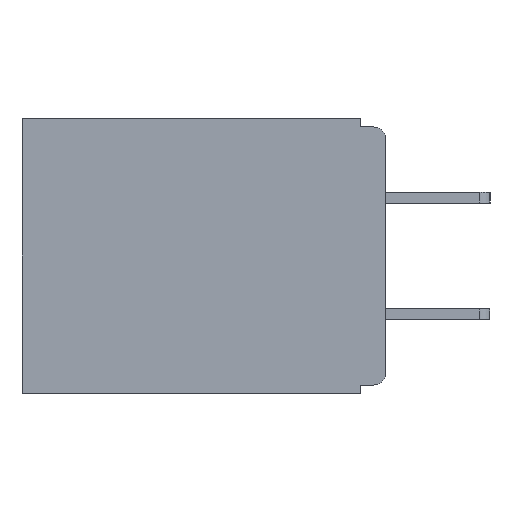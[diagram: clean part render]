
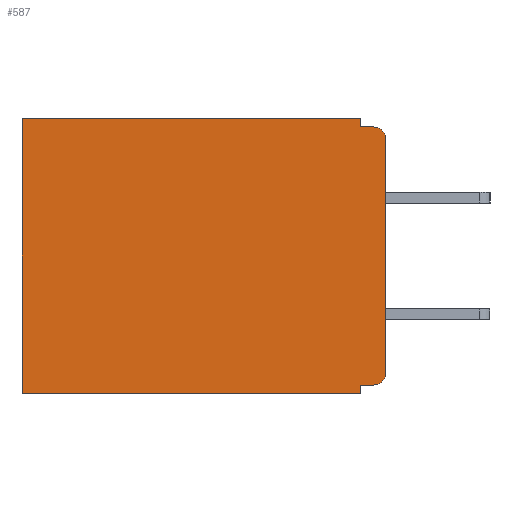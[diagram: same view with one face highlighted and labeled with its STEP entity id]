
A CAD part, left-side view. The second image highlights one B-rep face of the part: STEP entity #587.
In plain terms, the highlighted planar face has unit normal (-1, 0, 0).
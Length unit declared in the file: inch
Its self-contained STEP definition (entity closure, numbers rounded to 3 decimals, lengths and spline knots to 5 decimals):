
#24 = ORIENTED_EDGE ( 'NONE', *, *, #12456, .T. ) ;
#113 = EDGE_CURVE ( 'NONE', #2169, #9449, #17951, .T. ) ;
#400 = AXIS2_PLACEMENT_3D ( 'NONE', #11541, #19449, #19318 ) ;
#406 = CARTESIAN_POINT ( 'NONE',  ( 0.3, 0.031, 0. ) ) ;
#587 = ADVANCED_FACE ( 'NONE', ( #16894 ), #5696, .F. ) ;
#674 = LINE ( 'NONE', #2899, #17898 ) ;
#860 = VECTOR ( 'NONE', #5412, 39.37008 ) ;
#1231 = ORIENTED_EDGE ( 'NONE', *, *, #1955, .F. ) ;
#1410 = CARTESIAN_POINT ( 'NONE',  ( 0.3, 0.031, -0.01 ) ) ;
#1955 = EDGE_CURVE ( 'NONE', #13222, #3481, #2983, .T. ) ;
#2047 = CARTESIAN_POINT ( 'NONE',  ( 0.3, 0.031, -0.33 ) ) ;
#2169 = VERTEX_POINT ( 'NONE', #2966 ) ;
#2665 = CARTESIAN_POINT ( 'NONE',  ( 0.3, 0., -0.305 ) ) ;
#2899 = CARTESIAN_POINT ( 'NONE',  ( 0.3, 0., 0. ) ) ;
#2966 = CARTESIAN_POINT ( 'NONE',  ( 0.3, 0., -0.025 ) ) ;
#2983 = LINE ( 'NONE', #6736, #20175 ) ;
#3008 = ORIENTED_EDGE ( 'NONE', *, *, #3570, .T. ) ;
#3139 = EDGE_CURVE ( 'NONE', #14326, #16589, #4849, .T. ) ;
#3334 = DIRECTION ( 'NONE',  ( -1., 0., 0. ) ) ;
#3481 = VERTEX_POINT ( 'NONE', #20053 ) ;
#3570 = EDGE_CURVE ( 'NONE', #2169, #16589, #9251, .T. ) ;
#4005 = EDGE_CURVE ( 'NONE', #12849, #9449, #9772, .T. ) ;
#4008 = VECTOR ( 'NONE', #18722, 39.37008 ) ;
#4676 = VERTEX_POINT ( 'NONE', #406 ) ;
#4700 = EDGE_CURVE ( 'NONE', #18115, #13222, #18253, .T. ) ;
#4849 = LINE ( 'NONE', #18784, #9819 ) ;
#5397 = LINE ( 'NONE', #11966, #860 ) ;
#5410 = ORIENTED_EDGE ( 'NONE', *, *, #9202, .F. ) ;
#5412 = DIRECTION ( 'NONE',  ( 0., 0., -1. ) ) ;
#5484 = CARTESIAN_POINT ( 'NONE',  ( 0.3, 0., -0.32 ) ) ;
#5696 = PLANE ( 'NONE',  #400 ) ;
#6101 = ORIENTED_EDGE ( 'NONE', *, *, #3139, .F. ) ;
#6109 = CARTESIAN_POINT ( 'NONE',  ( 0.3, 0.015, -0.32 ) ) ;
#6736 = CARTESIAN_POINT ( 'NONE',  ( 0.3, 0., -0.33 ) ) ;
#6982 = EDGE_LOOP ( 'NONE', ( #16431, #3008, #6101, #16117, #24, #18254, #1231, #18808, #5410, #8944 ) ) ;
#7093 = CARTESIAN_POINT ( 'NONE',  ( 0.3, 0.031, -0.32 ) ) ;
#7620 = DIRECTION ( 'NONE',  ( -1., 0., 0. ) ) ;
#7667 = CARTESIAN_POINT ( 'NONE',  ( 0.3, 0.015, -0.305 ) ) ;
#7770 = CARTESIAN_POINT ( 'NONE',  ( 0.3, 0.015, -0.01 ) ) ;
#8492 = LINE ( 'NONE', #5484, #4008 ) ;
#8944 = ORIENTED_EDGE ( 'NONE', *, *, #4005, .T. ) ;
#9101 = EDGE_CURVE ( 'NONE', #18531, #3481, #19645, .T. ) ;
#9168 = EDGE_CURVE ( 'NONE', #4676, #14326, #5397, .T. ) ;
#9202 = EDGE_CURVE ( 'NONE', #12849, #18115, #8492, .T. ) ;
#9251 = CIRCLE ( 'NONE', #21141, 0.015 ) ;
#9449 = VERTEX_POINT ( 'NONE', #2665 ) ;
#9458 = CARTESIAN_POINT ( 'NONE',  ( 0.3, 0.015, -0.025 ) ) ;
#9686 = VECTOR ( 'NONE', #12217, 39.37008 ) ;
#9770 = DIRECTION ( 'NONE',  ( 0., 1., 0. ) ) ;
#9772 = CIRCLE ( 'NONE', #19671, 0.015 ) ;
#9819 = VECTOR ( 'NONE', #10908, 39.37008 ) ;
#10908 = DIRECTION ( 'NONE',  ( 0., -1., 0. ) ) ;
#11541 = CARTESIAN_POINT ( 'NONE',  ( 0.3, 0., -0.33 ) ) ;
#11760 = CARTESIAN_POINT ( 'NONE',  ( 0.3, 0.437, -0.33 ) ) ;
#11966 = CARTESIAN_POINT ( 'NONE',  ( 0.3, 0.031, 0. ) ) ;
#12217 = DIRECTION ( 'NONE',  ( 0., 0., -1. ) ) ;
#12286 = CARTESIAN_POINT ( 'NONE',  ( 0.3, 0., -0.33 ) ) ;
#12456 = EDGE_CURVE ( 'NONE', #4676, #18531, #674, .T. ) ;
#12789 = DIRECTION ( 'NONE',  ( 0., 1., 0. ) ) ;
#12849 = VERTEX_POINT ( 'NONE', #6109 ) ;
#13130 = CARTESIAN_POINT ( 'NONE',  ( 0.3, 0.437, 0. ) ) ;
#13222 = VERTEX_POINT ( 'NONE', #2047 ) ;
#13839 = VECTOR ( 'NONE', #21049, 39.37008 ) ;
#14326 = VERTEX_POINT ( 'NONE', #1410 ) ;
#15230 = VECTOR ( 'NONE', #16784, 39.37008 ) ;
#15950 = DIRECTION ( 'NONE',  ( 0., 0., -1. ) ) ;
#16117 = ORIENTED_EDGE ( 'NONE', *, *, #9168, .F. ) ;
#16431 = ORIENTED_EDGE ( 'NONE', *, *, #113, .F. ) ;
#16589 = VERTEX_POINT ( 'NONE', #7770 ) ;
#16718 = DIRECTION ( 'NONE',  ( 0., 0., -1. ) ) ;
#16784 = DIRECTION ( 'NONE',  ( 0., 0., -1. ) ) ;
#16894 = FACE_OUTER_BOUND ( 'NONE', #6982, .T. ) ;
#17898 = VECTOR ( 'NONE', #9770, 39.37008 ) ;
#17951 = LINE ( 'NONE', #12286, #9686 ) ;
#18115 = VERTEX_POINT ( 'NONE', #7093 ) ;
#18253 = LINE ( 'NONE', #18883, #13839 ) ;
#18254 = ORIENTED_EDGE ( 'NONE', *, *, #9101, .T. ) ;
#18531 = VERTEX_POINT ( 'NONE', #13130 ) ;
#18722 = DIRECTION ( 'NONE',  ( 0., 1., 0. ) ) ;
#18784 = CARTESIAN_POINT ( 'NONE',  ( 0.3, 0., -0.01 ) ) ;
#18808 = ORIENTED_EDGE ( 'NONE', *, *, #4700, .F. ) ;
#18883 = CARTESIAN_POINT ( 'NONE',  ( 0.3, 0.031, -0.33 ) ) ;
#19318 = DIRECTION ( 'NONE',  ( 0., 0., -1. ) ) ;
#19449 = DIRECTION ( 'NONE',  ( 1., 0., 0. ) ) ;
#19645 = LINE ( 'NONE', #11760, #15230 ) ;
#19671 = AXIS2_PLACEMENT_3D ( 'NONE', #7667, #3334, #15950 ) ;
#20053 = CARTESIAN_POINT ( 'NONE',  ( 0.3, 0.437, -0.33 ) ) ;
#20175 = VECTOR ( 'NONE', #12789, 39.37008 ) ;
#21049 = DIRECTION ( 'NONE',  ( 0., 0., -1. ) ) ;
#21141 = AXIS2_PLACEMENT_3D ( 'NONE', #9458, #7620, #16718 ) ;
